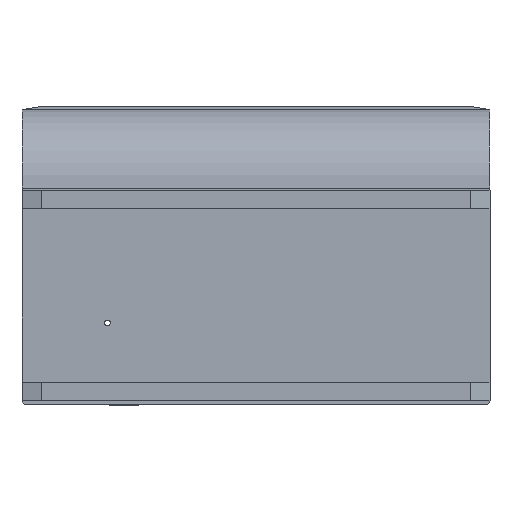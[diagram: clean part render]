
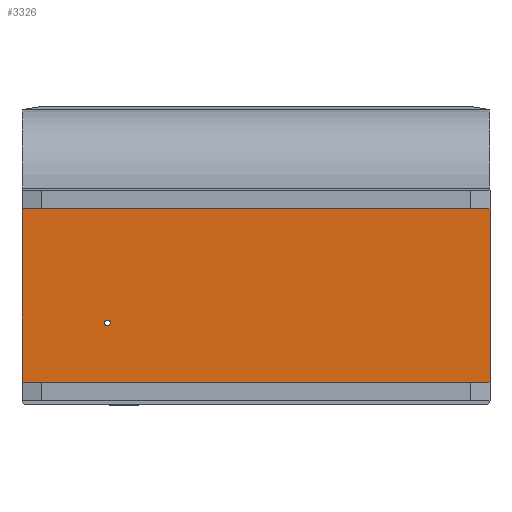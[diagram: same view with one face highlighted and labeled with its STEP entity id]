
A CAD part, top view. The second image highlights one B-rep face of the part: STEP entity #3326.
In plain terms, the highlighted planar face has unit normal (0, 0, 1).
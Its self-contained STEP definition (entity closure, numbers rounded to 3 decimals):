
#34 = EDGE_LOOP ( 'NONE', ( #3798, #3226, #950, #46 ) ) ;
#46 = ORIENTED_EDGE ( 'NONE', *, *, #504, .F. ) ;
#59 = VECTOR ( 'NONE', #4265, 1000. ) ;
#128 = CARTESIAN_POINT ( 'NONE',  ( -21.21, 13.639, 13.681 ) ) ;
#288 = CARTESIAN_POINT ( 'NONE',  ( -21.21, 44.495, 13.681 ) ) ;
#307 = DIRECTION ( 'NONE',  ( 0., 1., 0. ) ) ;
#451 = DIRECTION ( 'NONE',  ( 0., 1., 0. ) ) ;
#504 = EDGE_CURVE ( 'NONE', #862, #3507, #2292, .T. ) ;
#689 = CARTESIAN_POINT ( 'NONE',  ( -98.399, 15.895, 13.681 ) ) ;
#765 = CARTESIAN_POINT ( 'NONE',  ( -97.21, 15.895, 13.681 ) ) ;
#862 = VERTEX_POINT ( 'NONE', #288 ) ;
#950 = ORIENTED_EDGE ( 'NONE', *, *, #3133, .T. ) ;
#1063 = ORIENTED_EDGE ( 'NONE', *, *, #4460, .F. ) ;
#1267 = EDGE_LOOP ( 'NONE', ( #1063 ) ) ;
#1337 = DIRECTION ( 'NONE',  ( 0., 0., -1. ) ) ;
#1395 = LINE ( 'NONE', #765, #59 ) ;
#1536 = CARTESIAN_POINT ( 'NONE',  ( -98.399, 28.911, 13.681 ) ) ;
#1589 = CARTESIAN_POINT ( 'NONE',  ( -98.399, 44.495, 13.681 ) ) ;
#1621 = DIRECTION ( 'NONE',  ( -1., 0., 0. ) ) ;
#1760 = CIRCLE ( 'NONE', #4280, 0.484 ) ;
#1791 = FACE_OUTER_BOUND ( 'NONE', #34, .T. ) ;
#1887 = DIRECTION ( 'NONE',  ( 0., -1., 0. ) ) ;
#2055 = DIRECTION ( 'NONE',  ( 0., 0., 1. ) ) ;
#2153 = FACE_BOUND ( 'NONE', #1267, .T. ) ;
#2292 = LINE ( 'NONE', #128, #3932 ) ;
#2798 = CARTESIAN_POINT ( 'NONE',  ( -21.21, 15.895, 13.681 ) ) ;
#2805 = LINE ( 'NONE', #1536, #3021 ) ;
#3021 = VECTOR ( 'NONE', #451, 1000. ) ;
#3133 = EDGE_CURVE ( 'NONE', #4546, #3507, #1395, .T. ) ;
#3135 = CARTESIAN_POINT ( 'NONE',  ( -84.335, 26.135, 13.681 ) ) ;
#3226 = ORIENTED_EDGE ( 'NONE', *, *, #3575, .F. ) ;
#3319 = CARTESIAN_POINT ( 'NONE',  ( -22.21, 44.495, 13.681 ) ) ;
#3326 = ADVANCED_FACE ( 'NONE', ( #1791, #2153 ), #4188, .F. ) ;
#3420 = VERTEX_POINT ( 'NONE', #3135 ) ;
#3507 = VERTEX_POINT ( 'NONE', #2798 ) ;
#3575 = EDGE_CURVE ( 'NONE', #4546, #4213, #2805, .T. ) ;
#3798 = ORIENTED_EDGE ( 'NONE', *, *, #4170, .T. ) ;
#3811 = DIRECTION ( 'NONE',  ( 0., 1., 0. ) ) ;
#3929 = AXIS2_PLACEMENT_3D ( 'NONE', #4534, #1337, #3811 ) ;
#3932 = VECTOR ( 'NONE', #1887, 1000. ) ;
#3995 = LINE ( 'NONE', #3319, #4161 ) ;
#4161 = VECTOR ( 'NONE', #1621, 1000. ) ;
#4170 = EDGE_CURVE ( 'NONE', #862, #4213, #3995, .T. ) ;
#4188 = PLANE ( 'NONE',  #3929 ) ;
#4213 = VERTEX_POINT ( 'NONE', #1589 ) ;
#4265 = DIRECTION ( 'NONE',  ( 1., 0., 0. ) ) ;
#4280 = AXIS2_PLACEMENT_3D ( 'NONE', #4475, #2055, #307 ) ;
#4460 = EDGE_CURVE ( 'NONE', #3420, #3420, #1760, .T. ) ;
#4475 = CARTESIAN_POINT ( 'NONE',  ( -84.335, 25.651, 13.681 ) ) ;
#4534 = CARTESIAN_POINT ( 'NONE',  ( -21.21, 12.227, 13.681 ) ) ;
#4546 = VERTEX_POINT ( 'NONE', #689 ) ;
